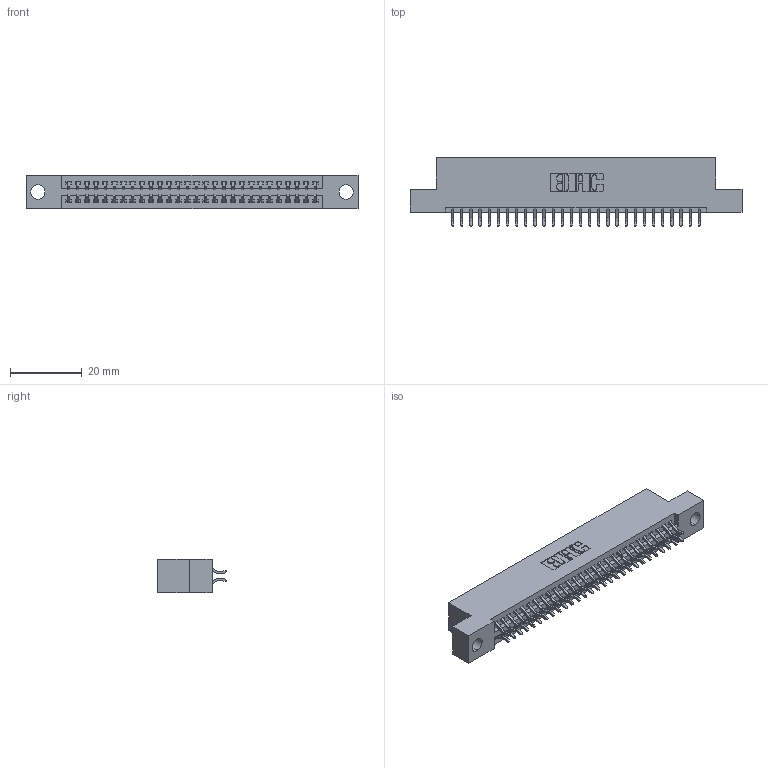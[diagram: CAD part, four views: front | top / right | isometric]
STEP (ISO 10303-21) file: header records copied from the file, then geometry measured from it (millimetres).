
FILE_DESCRIPTION (( 'STEP AP203' ), '1' );
FILE_NAME ('395-056-556-204.STEP', '2021-06-17T01:18:03', ( '' ), ( '' ), 'SwSTEP 2.0', 'SolidWorks 2020', '' );
FILE_SCHEMA (( 'CONFIG_CONTROL_DESIGN' ));
Length unit declared in the file: inch
Products named in the file (3): 345 Part_Flush Mounting Lugs - 0.156 Dia-TI; 345-292-001_556 Tail; 395-056-556-204
Assembly tree (57 placements, depth 2):
  395-056-556-204
    345 Part_Flush Mounting Lugs - 0.156 Dia-TI
    345-292-001_556 Tail  x56
Bounding box: 92.33 x 19.24 x 9.4 mm (x, y, z)
Volume: 8730.8 mm3; surface area: 12437 mm2
Topology: 57 solids, 57 shells, 3276 faces, 9729 edges, 6410 vertices
Faces by surface type: plane 2166, cylinder 1110
Entity records: 24493 total; most frequent: CARTESIAN_POINT 4138, ORIENTED_EDGE 4058, DIRECTION 3653, EDGE_CURVE 2029, VECTOR 1777, LINE 1777, VERTEX_POINT 1350, AXIS2_PLACEMENT_3D 938
